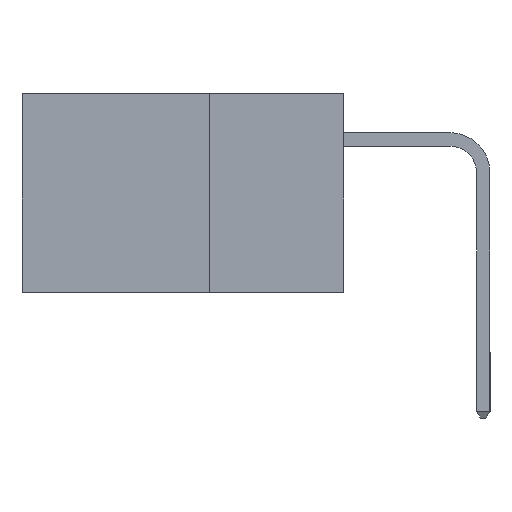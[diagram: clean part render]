
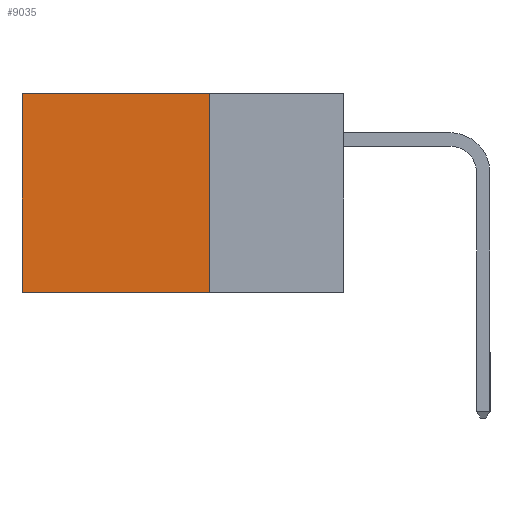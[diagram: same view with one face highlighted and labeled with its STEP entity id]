
A CAD part, left-side view. The second image highlights one B-rep face of the part: STEP entity #9035.
In plain terms, the highlighted planar face has unit normal (-1, 0, 0).
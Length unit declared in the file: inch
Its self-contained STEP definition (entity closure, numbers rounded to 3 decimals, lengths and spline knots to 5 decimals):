
#450 = FACE_OUTER_BOUND ( 'NONE', #10470, .T. ) ;
#654 = LINE ( 'NONE', #6125, #10444 ) ;
#869 = ORIENTED_EDGE ( 'NONE', *, *, #1347, .F. ) ;
#1305 = DIRECTION ( 'NONE',  ( 0., 0., -1. ) ) ;
#1347 = EDGE_CURVE ( 'NONE', #5857, #2403, #12207, .T. ) ;
#1477 = CARTESIAN_POINT ( 'NONE',  ( 0.298, 0.25, 0. ) ) ;
#1602 = CARTESIAN_POINT ( 'NONE',  ( 0.298, 0.25, 0. ) ) ;
#1687 = DIRECTION ( 'NONE',  ( 0., 0., -1. ) ) ;
#1691 = VERTEX_POINT ( 'NONE', #10384 ) ;
#2403 = VERTEX_POINT ( 'NONE', #8476 ) ;
#3094 = VECTOR ( 'NONE', #8928, 39.37008 ) ;
#3395 = CARTESIAN_POINT ( 'NONE',  ( 0.298, 0.25, -0.37 ) ) ;
#3416 = LINE ( 'NONE', #12039, #3094 ) ;
#4655 = ORIENTED_EDGE ( 'NONE', *, *, #8991, .F. ) ;
#5459 = ORIENTED_EDGE ( 'NONE', *, *, #7704, .T. ) ;
#5680 = PLANE ( 'NONE',  #5995 ) ;
#5857 = VERTEX_POINT ( 'NONE', #6834 ) ;
#5995 = AXIS2_PLACEMENT_3D ( 'NONE', #1602, #11618, #1687 ) ;
#6125 = CARTESIAN_POINT ( 'NONE',  ( 0.298, 0.6, 0. ) ) ;
#6834 = CARTESIAN_POINT ( 'NONE',  ( 0.298, 0.25, -0.37 ) ) ;
#7376 = VECTOR ( 'NONE', #12208, 39.37008 ) ;
#7610 = VECTOR ( 'NONE', #8432, 39.37008 ) ;
#7704 = EDGE_CURVE ( 'NONE', #9429, #1691, #3416, .T. ) ;
#8432 = DIRECTION ( 'NONE',  ( 0., 0., -1. ) ) ;
#8476 = CARTESIAN_POINT ( 'NONE',  ( 0.298, 0.6, -0.37 ) ) ;
#8928 = DIRECTION ( 'NONE',  ( 0., 1., 0. ) ) ;
#8991 = EDGE_CURVE ( 'NONE', #9429, #5857, #12139, .T. ) ;
#9035 = ADVANCED_FACE ( 'NONE', ( #450 ), #5680, .F. ) ;
#9429 = VERTEX_POINT ( 'NONE', #10188 ) ;
#10188 = CARTESIAN_POINT ( 'NONE',  ( 0.298, 0.25, 0. ) ) ;
#10384 = CARTESIAN_POINT ( 'NONE',  ( 0.298, 0.6, 0. ) ) ;
#10444 = VECTOR ( 'NONE', #1305, 39.37008 ) ;
#10470 = EDGE_LOOP ( 'NONE', ( #12678, #869, #4655, #5459 ) ) ;
#11261 = EDGE_CURVE ( 'NONE', #1691, #2403, #654, .T. ) ;
#11618 = DIRECTION ( 'NONE',  ( 1., 0., 0. ) ) ;
#12039 = CARTESIAN_POINT ( 'NONE',  ( 0.298, 0.25, 0. ) ) ;
#12139 = LINE ( 'NONE', #1477, #7610 ) ;
#12207 = LINE ( 'NONE', #3395, #7376 ) ;
#12208 = DIRECTION ( 'NONE',  ( 0., 1., 0. ) ) ;
#12678 = ORIENTED_EDGE ( 'NONE', *, *, #11261, .T. ) ;
